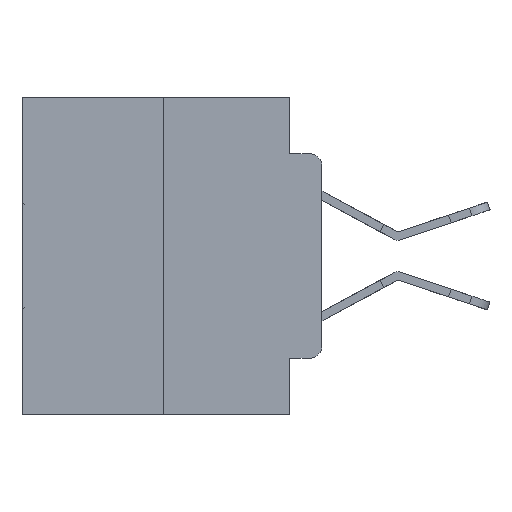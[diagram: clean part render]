
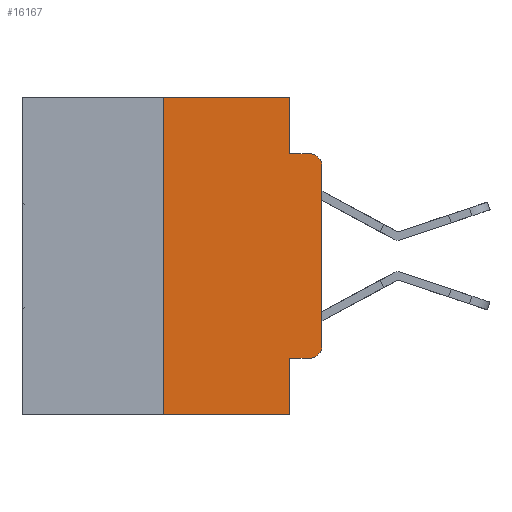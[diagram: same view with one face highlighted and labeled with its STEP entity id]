
A CAD part, left-side view. The second image highlights one B-rep face of the part: STEP entity #16167.
In plain terms, the highlighted planar face has unit normal (-1, 0, 0).
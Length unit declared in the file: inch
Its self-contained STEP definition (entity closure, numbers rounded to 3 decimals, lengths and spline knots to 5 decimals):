
#7 = DIRECTION ( 'NONE',  ( 0., -1., 0. ) ) ;
#71 = CARTESIAN_POINT ( 'NONE',  ( 0., 0.473, 0. ) ) ;
#541 = AXIS2_PLACEMENT_3D ( 'NONE', #17826, #3434, #20231 ) ;
#1434 = EDGE_CURVE ( 'NONE', #10499, #26913, #22465, .T. ) ;
#1505 = EDGE_CURVE ( 'NONE', #2192, #26104, #14570, .T. ) ;
#1630 = VECTOR ( 'NONE', #22177, 39.37008 ) ;
#1814 = EDGE_LOOP ( 'NONE', ( #12041, #13543, #14282, #3018, #28504, #29226, #30714, #18803, #9034, #4889 ) ) ;
#1932 = AXIS2_PLACEMENT_3D ( 'NONE', #16422, #2049, #18837 ) ;
#2049 = DIRECTION ( 'NONE',  ( -1., 0., 0. ) ) ;
#2192 = VERTEX_POINT ( 'NONE', #7350 ) ;
#2500 = DIRECTION ( 'NONE',  ( 1., 0., 0. ) ) ;
#2674 = CARTESIAN_POINT ( 'NONE',  ( 0., 0.02, -0.0885 ) ) ;
#3018 = ORIENTED_EDGE ( 'NONE', *, *, #7903, .F. ) ;
#3434 = DIRECTION ( 'NONE',  ( -1., 0., 0. ) ) ;
#3536 = DIRECTION ( 'NONE',  ( 0., 0., -1. ) ) ;
#3623 = LINE ( 'NONE', #17933, #9260 ) ;
#3659 = LINE ( 'NONE', #21639, #9297 ) ;
#4324 = CARTESIAN_POINT ( 'NONE',  ( 0., 0.051, -0.0885 ) ) ;
#4889 = ORIENTED_EDGE ( 'NONE', *, *, #21729, .T. ) ;
#5183 = VERTEX_POINT ( 'NONE', #18162 ) ;
#6901 = CARTESIAN_POINT ( 'NONE',  ( 0., 0.051, -0.4115 ) ) ;
#7350 = CARTESIAN_POINT ( 'NONE',  ( 0., 0.25, -0.5 ) ) ;
#7903 = EDGE_CURVE ( 'NONE', #15311, #10499, #19129, .T. ) ;
#9001 = DIRECTION ( 'NONE',  ( 0., 0., -1. ) ) ;
#9016 = CARTESIAN_POINT ( 'NONE',  ( 0., 0.25, 0. ) ) ;
#9034 = ORIENTED_EDGE ( 'NONE', *, *, #20490, .T. ) ;
#9128 = CARTESIAN_POINT ( 'NONE',  ( 0., 0.051, -0.5 ) ) ;
#9260 = VECTOR ( 'NONE', #3536, 39.37008 ) ;
#9297 = VECTOR ( 'NONE', #7, 39.37008 ) ;
#9603 = EDGE_CURVE ( 'NONE', #29944, #27921, #3623, .T. ) ;
#10499 = VERTEX_POINT ( 'NONE', #4324 ) ;
#12041 = ORIENTED_EDGE ( 'NONE', *, *, #14031, .T. ) ;
#12061 = CARTESIAN_POINT ( 'NONE',  ( 0., 0.25, 0. ) ) ;
#12889 = LINE ( 'NONE', #26962, #1630 ) ;
#13543 = ORIENTED_EDGE ( 'NONE', *, *, #23333, .T. ) ;
#14031 = EDGE_CURVE ( 'NONE', #26634, #16199, #12889, .T. ) ;
#14261 = VECTOR ( 'NONE', #9001, 39.37008 ) ;
#14282 = ORIENTED_EDGE ( 'NONE', *, *, #1434, .F. ) ;
#14284 = AXIS2_PLACEMENT_3D ( 'NONE', #71, #2500, #19288 ) ;
#14305 = FACE_OUTER_BOUND ( 'NONE', #1814, .T. ) ;
#14456 = DIRECTION ( 'NONE',  ( 0., 0., 1. ) ) ;
#14458 = PLANE ( 'NONE',  #14284 ) ;
#14570 = LINE ( 'NONE', #12061, #27294 ) ;
#15311 = VERTEX_POINT ( 'NONE', #28006 ) ;
#16099 = VECTOR ( 'NONE', #18969, 39.37008 ) ;
#16167 = ADVANCED_FACE ( 'NONE', ( #14305 ), #14458, .F. ) ;
#16199 = VERTEX_POINT ( 'NONE', #21695 ) ;
#16422 = CARTESIAN_POINT ( 'NONE',  ( 0., 0.02, -0.3915 ) ) ;
#16562 = CARTESIAN_POINT ( 'NONE',  ( 0., 0.051, -0.0885 ) ) ;
#17826 = CARTESIAN_POINT ( 'NONE',  ( 0., 0.02, -0.1085 ) ) ;
#17933 = CARTESIAN_POINT ( 'NONE',  ( 0., 0.051, 0. ) ) ;
#18067 = LINE ( 'NONE', #6901, #24446 ) ;
#18162 = CARTESIAN_POINT ( 'NONE',  ( 0., 0.02, -0.4115 ) ) ;
#18803 = ORIENTED_EDGE ( 'NONE', *, *, #9603, .F. ) ;
#18837 = DIRECTION ( 'NONE',  ( 0., 0., -1. ) ) ;
#18969 = DIRECTION ( 'NONE',  ( 0., -1., 0. ) ) ;
#19129 = LINE ( 'NONE', #20981, #14261 ) ;
#19288 = DIRECTION ( 'NONE',  ( 0., 0., -1. ) ) ;
#20231 = DIRECTION ( 'NONE',  ( 0., 0., -1. ) ) ;
#20490 = EDGE_CURVE ( 'NONE', #29944, #5183, #18067, .T. ) ;
#20981 = CARTESIAN_POINT ( 'NONE',  ( 0., 0.051, 0. ) ) ;
#21263 = CIRCLE ( 'NONE', #541, 0.02 ) ;
#21268 = VECTOR ( 'NONE', #26073, 39.37008 ) ;
#21326 = DIRECTION ( 'NONE',  ( 0., -1., 0. ) ) ;
#21639 = CARTESIAN_POINT ( 'NONE',  ( 0., 0.473, 0. ) ) ;
#21695 = CARTESIAN_POINT ( 'NONE',  ( 0., 0., -0.1085 ) ) ;
#21729 = EDGE_CURVE ( 'NONE', #5183, #26634, #28079, .T. ) ;
#22177 = DIRECTION ( 'NONE',  ( 0., 0., 1. ) ) ;
#22409 = EDGE_CURVE ( 'NONE', #26104, #15311, #3659, .T. ) ;
#22465 = LINE ( 'NONE', #16562, #16099 ) ;
#23333 = EDGE_CURVE ( 'NONE', #16199, #26913, #21263, .T. ) ;
#24446 = VECTOR ( 'NONE', #21326, 39.37008 ) ;
#25428 = EDGE_CURVE ( 'NONE', #2192, #27921, #28354, .T. ) ;
#25619 = CARTESIAN_POINT ( 'NONE',  ( 0., 0.051, -0.4115 ) ) ;
#26073 = DIRECTION ( 'NONE',  ( 0., -1., 0. ) ) ;
#26104 = VERTEX_POINT ( 'NONE', #9016 ) ;
#26634 = VERTEX_POINT ( 'NONE', #30312 ) ;
#26913 = VERTEX_POINT ( 'NONE', #2674 ) ;
#26962 = CARTESIAN_POINT ( 'NONE',  ( 0., 0., 0. ) ) ;
#27294 = VECTOR ( 'NONE', #14456, 39.37008 ) ;
#27921 = VERTEX_POINT ( 'NONE', #9128 ) ;
#28006 = CARTESIAN_POINT ( 'NONE',  ( 0., 0.051, 0. ) ) ;
#28079 = CIRCLE ( 'NONE', #1932, 0.02 ) ;
#28354 = LINE ( 'NONE', #30718, #21268 ) ;
#28504 = ORIENTED_EDGE ( 'NONE', *, *, #22409, .F. ) ;
#29226 = ORIENTED_EDGE ( 'NONE', *, *, #1505, .F. ) ;
#29944 = VERTEX_POINT ( 'NONE', #25619 ) ;
#30312 = CARTESIAN_POINT ( 'NONE',  ( 0., 0., -0.3915 ) ) ;
#30714 = ORIENTED_EDGE ( 'NONE', *, *, #25428, .T. ) ;
#30718 = CARTESIAN_POINT ( 'NONE',  ( 0., 0.473, -0.5 ) ) ;
